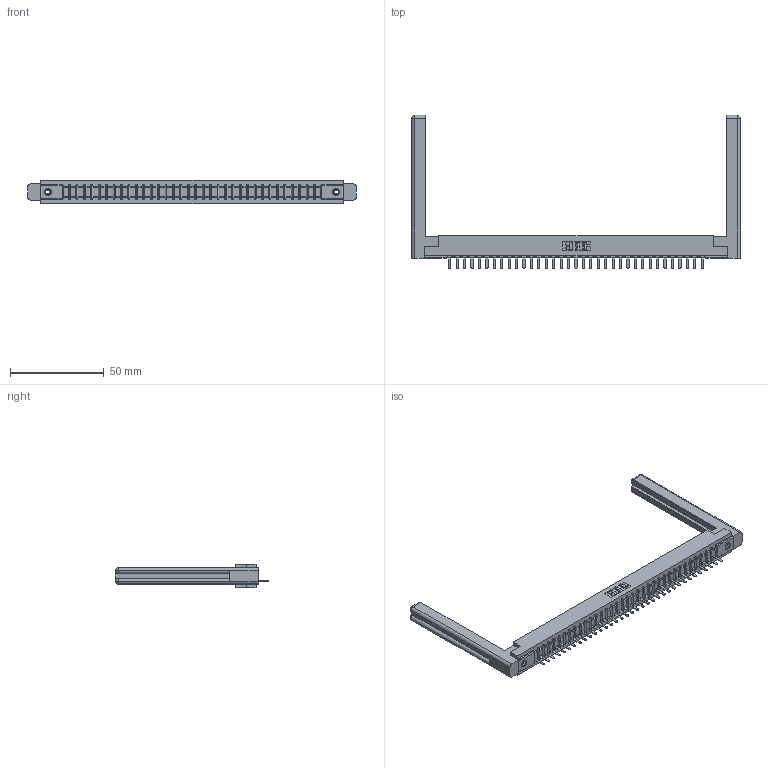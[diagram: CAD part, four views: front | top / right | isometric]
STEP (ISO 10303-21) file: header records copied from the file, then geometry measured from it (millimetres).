
FILE_DESCRIPTION (( 'STEP AP203' ), '1' );
FILE_NAME ('357-035-421-158.STEP', '2020-10-02T13:06:36', ( '' ), ( '' ), 'SwSTEP 2.0', 'SolidWorks 2020', '' );
FILE_SCHEMA (( 'CONFIG_CONTROL_DESIGN' ));
Length unit declared in the file: inch
Products named in the file (5): 307 Part_.156 Dia Mounting Holes; 345-250-001_345-250-001-102; 357-035-421-158; 307-220-058; 307-290-002_521
Assembly tree (40 placements, depth 2):
  357-035-421-158
    307 Part_.156 Dia Mounting Holes
    307-290-002_521  x35
    307-220-058  x2
    345-250-001_345-250-001-102  x2
Bounding box: 175.31 x 81.74 x 12.7 mm (x, y, z)
Volume: 25830.6 mm3; surface area: 28210 mm2
Topology: 40 solids, 40 shells, 2886 faces, 8797 edges, 5754 vertices
Faces by surface type: plane 1729, cylinder 1061, sphere 72, torus 12, cone 12
Entity records: 34219 total; most frequent: CARTESIAN_POINT 5779, ORIENTED_EDGE 5708, DIRECTION 5578, EDGE_CURVE 2854, LINE 2180, VECTOR 2180, VERTEX_POINT 1846, AXIS2_PLACEMENT_3D 1699
